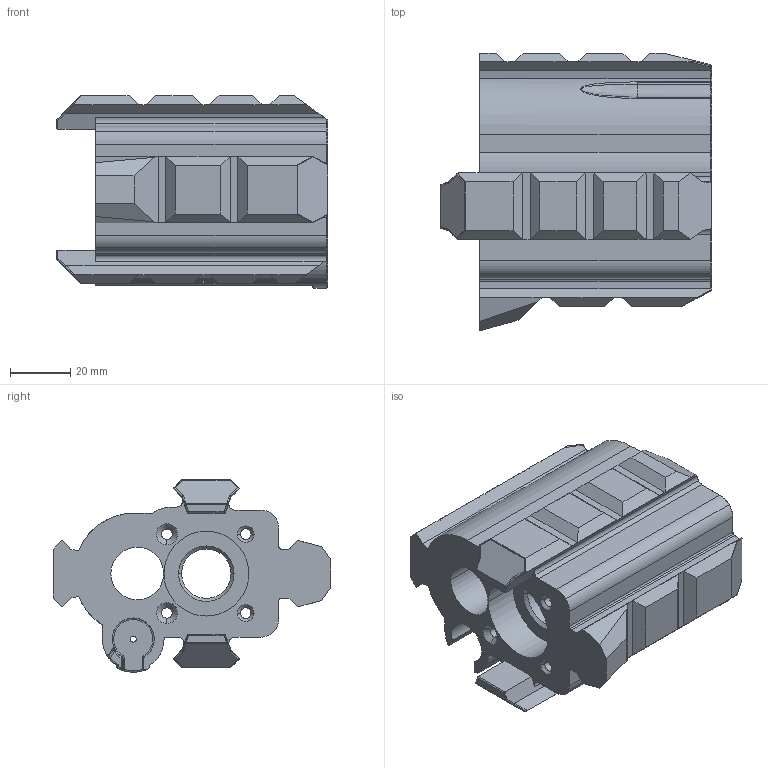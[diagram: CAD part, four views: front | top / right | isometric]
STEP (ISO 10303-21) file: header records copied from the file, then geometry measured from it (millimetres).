
FILE_DESCRIPTION(('STEP AP214'),'1');
FILE_NAME('MOD9E_barrel_retainer.stp','2020-09-01T22:15:27',(' '),(' '),'Spatial InterOp 3D',' ',' ');
FILE_SCHEMA(('AUTOMOTIVE_DESIGN { 1 0 10303 214 1 1 1 1 }'));
Length unit declared in the file: metre
Products named in the file (1): ASM Body
Bounding box: 90.02 x 92.13 x 63.85 mm (x, y, z)
Volume: 149392.5 mm3; surface area: 45969.4 mm2
Topology: 1 solids, 1 shells, 425 faces, 1093 edges, 668 vertices
Faces by surface type: plane 158, cylinder 152, cone 81, bspline 13, sphere 11, torus 10
Entity records: 15065 total; most frequent: CARTESIAN_POINT 4595, DIRECTION 2259, ORIENTED_EDGE 2178, EDGE_CURVE 1089, AXIS2_PLACEMENT_3D 826, VERTEX_POINT 668, LINE 607, VECTOR 607
